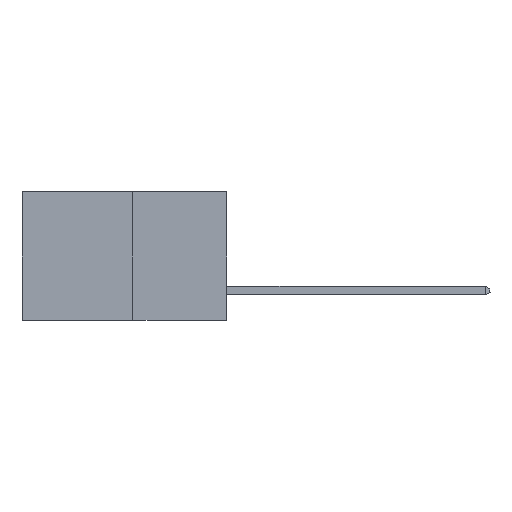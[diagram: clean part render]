
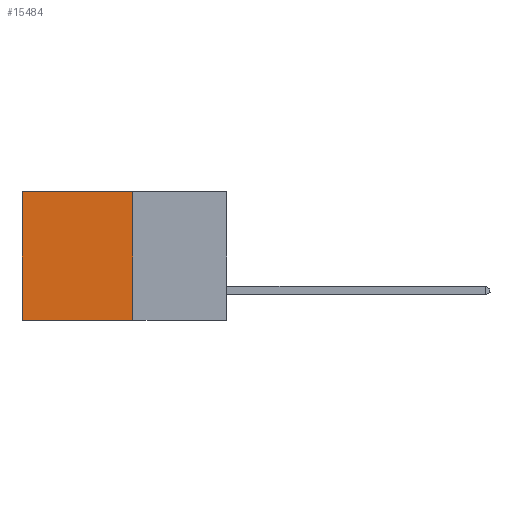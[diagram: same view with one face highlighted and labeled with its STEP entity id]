
A CAD part, left-side view. The second image highlights one B-rep face of the part: STEP entity #15484.
In plain terms, the highlighted planar face has unit normal (-1, 0, 0).
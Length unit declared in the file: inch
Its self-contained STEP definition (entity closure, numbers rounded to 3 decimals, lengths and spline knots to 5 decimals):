
#178 = LINE ( 'NONE', #3980, #2691 ) ;
#303 = DIRECTION ( 'NONE',  ( 0., 1., 0. ) ) ;
#385 = LINE ( 'NONE', #15459, #9796 ) ;
#686 = CARTESIAN_POINT ( 'NONE',  ( 0.277, 0.27, -0.37 ) ) ;
#858 = DIRECTION ( 'NONE',  ( 0., 0., -1. ) ) ;
#1200 = AXIS2_PLACEMENT_3D ( 'NONE', #6582, #10263, #2906 ) ;
#1659 = PLANE ( 'NONE',  #1200 ) ;
#2214 = LINE ( 'NONE', #2545, #14432 ) ;
#2545 = CARTESIAN_POINT ( 'NONE',  ( 0.277, 0.27, -0.37 ) ) ;
#2546 = VERTEX_POINT ( 'NONE', #686 ) ;
#2691 = VECTOR ( 'NONE', #303, 39.37008 ) ;
#2855 = CARTESIAN_POINT ( 'NONE',  ( 0.277, 0.59, -0.37 ) ) ;
#2906 = DIRECTION ( 'NONE',  ( 0., 0., -1. ) ) ;
#3322 = CARTESIAN_POINT ( 'NONE',  ( 0.277, 0.27, 0. ) ) ;
#3720 = ORIENTED_EDGE ( 'NONE', *, *, #14741, .F. ) ;
#3956 = ORIENTED_EDGE ( 'NONE', *, *, #11787, .T. ) ;
#3980 = CARTESIAN_POINT ( 'NONE',  ( 0.277, 0.27, -0.37 ) ) ;
#4232 = FACE_OUTER_BOUND ( 'NONE', #6696, .T. ) ;
#5392 = DIRECTION ( 'NONE',  ( 0., 1., 0. ) ) ;
#6528 = VERTEX_POINT ( 'NONE', #14006 ) ;
#6582 = CARTESIAN_POINT ( 'NONE',  ( 0.277, 0.27, -0.37 ) ) ;
#6696 = EDGE_LOOP ( 'NONE', ( #13881, #3720, #8732, #3956 ) ) ;
#7009 = LINE ( 'NONE', #10256, #13096 ) ;
#8028 = EDGE_CURVE ( 'NONE', #10349, #2546, #2214, .T. ) ;
#8670 = DIRECTION ( 'NONE',  ( 0., 0., -1. ) ) ;
#8732 = ORIENTED_EDGE ( 'NONE', *, *, #8028, .F. ) ;
#9796 = VECTOR ( 'NONE', #858, 39.37008 ) ;
#10256 = CARTESIAN_POINT ( 'NONE',  ( 0.277, 0.27, 0. ) ) ;
#10263 = DIRECTION ( 'NONE',  ( 1., 0., 0. ) ) ;
#10349 = VERTEX_POINT ( 'NONE', #3322 ) ;
#11787 = EDGE_CURVE ( 'NONE', #10349, #6528, #7009, .T. ) ;
#13096 = VECTOR ( 'NONE', #5392, 39.37008 ) ;
#13871 = EDGE_CURVE ( 'NONE', #6528, #15465, #385, .T. ) ;
#13881 = ORIENTED_EDGE ( 'NONE', *, *, #13871, .T. ) ;
#14006 = CARTESIAN_POINT ( 'NONE',  ( 0.277, 0.59, 0. ) ) ;
#14432 = VECTOR ( 'NONE', #8670, 39.37008 ) ;
#14741 = EDGE_CURVE ( 'NONE', #2546, #15465, #178, .T. ) ;
#15459 = CARTESIAN_POINT ( 'NONE',  ( 0.277, 0.59, -0.37 ) ) ;
#15465 = VERTEX_POINT ( 'NONE', #2855 ) ;
#15484 = ADVANCED_FACE ( 'NONE', ( #4232 ), #1659, .F. ) ;
